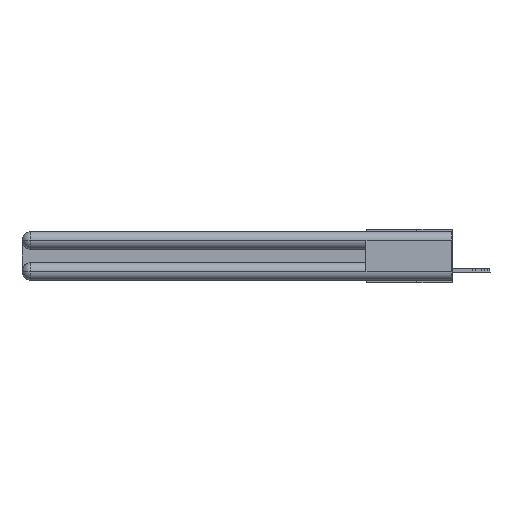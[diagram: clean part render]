
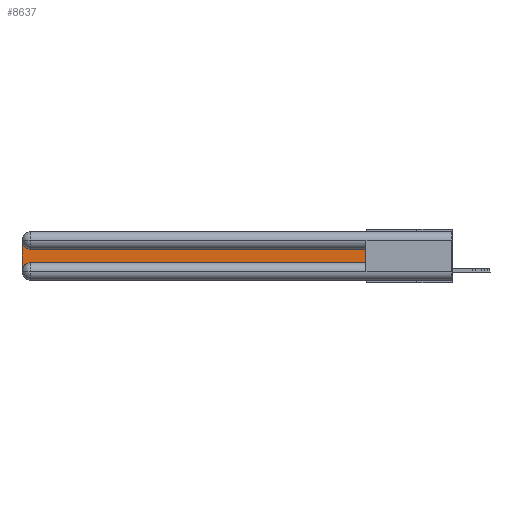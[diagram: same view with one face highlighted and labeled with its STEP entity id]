
A CAD part, left-side view. The second image highlights one B-rep face of the part: STEP entity #8637.
In plain terms, the highlighted planar face has unit normal (-1, 0, 0).
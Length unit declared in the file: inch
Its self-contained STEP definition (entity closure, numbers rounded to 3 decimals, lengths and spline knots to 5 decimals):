
#626 = ORIENTED_EDGE ( 'NONE', *, *, #10922, .T. ) ;
#1539 = DIRECTION ( 'NONE',  ( 1., 0., 0. ) ) ;
#1591 = AXIS2_PLACEMENT_3D ( 'NONE', #20663, #12597, #2594 ) ;
#2594 = DIRECTION ( 'NONE',  ( 0., 0., -1. ) ) ;
#2846 = CARTESIAN_POINT ( 'NONE',  ( 0.075, 0.6, -0.2175 ) ) ;
#2867 = EDGE_CURVE ( 'NONE', #4830, #20696, #9017, .T. ) ;
#3170 = DIRECTION ( 'NONE',  ( 0., 0., -1. ) ) ;
#4822 = VECTOR ( 'NONE', #10806, 39.37008 ) ;
#4830 = VERTEX_POINT ( 'NONE', #29184 ) ;
#4852 = ORIENTED_EDGE ( 'NONE', *, *, #13055, .T. ) ;
#5380 = VECTOR ( 'NONE', #6955, 39.37008 ) ;
#5693 = VERTEX_POINT ( 'NONE', #28996 ) ;
#5864 = VECTOR ( 'NONE', #19027, 39.37008 ) ;
#6955 = DIRECTION ( 'NONE',  ( 0., 0., 1. ) ) ;
#6956 = AXIS2_PLACEMENT_3D ( 'NONE', #14237, #1539, #21978 ) ;
#8501 = CARTESIAN_POINT ( 'NONE',  ( 0.075, 0.6, -0.1225 ) ) ;
#8637 = ADVANCED_FACE ( 'NONE', ( #25916 ), #29512, .F. ) ;
#9017 = LINE ( 'NONE', #8501, #5864 ) ;
#9150 = LINE ( 'NONE', #2846, #4822 ) ;
#9892 = VERTEX_POINT ( 'NONE', #15223 ) ;
#10806 = DIRECTION ( 'NONE',  ( 0., -1., 0. ) ) ;
#10922 = EDGE_CURVE ( 'NONE', #30947, #4830, #32181, .T. ) ;
#11795 = CIRCLE ( 'NONE', #1591, 0.06 ) ;
#12597 = DIRECTION ( 'NONE',  ( 1., 0., 0. ) ) ;
#13055 = EDGE_CURVE ( 'NONE', #20696, #5693, #21182, .T. ) ;
#13077 = EDGE_CURVE ( 'NONE', #26933, #30947, #9150, .T. ) ;
#13784 = ORIENTED_EDGE ( 'NONE', *, *, #2867, .T. ) ;
#14237 = CARTESIAN_POINT ( 'NONE',  ( 0.075, 3., -0.1225 ) ) ;
#14906 = CARTESIAN_POINT ( 'NONE',  ( 0.075, 0.6, -0.2175 ) ) ;
#15223 = CARTESIAN_POINT ( 'NONE',  ( 0.075, 3., -0.2775 ) ) ;
#15667 = CARTESIAN_POINT ( 'NONE',  ( 0.075, 2.94, -0.2175 ) ) ;
#18065 = EDGE_CURVE ( 'NONE', #9892, #26933, #11795, .T. ) ;
#19027 = DIRECTION ( 'NONE',  ( 0., 1., 0. ) ) ;
#20663 = CARTESIAN_POINT ( 'NONE',  ( 0.075, 2.94, -0.2775 ) ) ;
#20696 = VERTEX_POINT ( 'NONE', #24758 ) ;
#21182 = CIRCLE ( 'NONE', #26749, 0.06 ) ;
#21938 = CARTESIAN_POINT ( 'NONE',  ( 0.075, 0.6, -0.2175 ) ) ;
#21978 = DIRECTION ( 'NONE',  ( 0., 0., -1. ) ) ;
#23483 = DIRECTION ( 'NONE',  ( 1., 0., 0. ) ) ;
#24049 = ORIENTED_EDGE ( 'NONE', *, *, #18065, .T. ) ;
#24758 = CARTESIAN_POINT ( 'NONE',  ( 0.075, 2.94, -0.1225 ) ) ;
#24903 = EDGE_LOOP ( 'NONE', ( #13784, #4852, #27246, #24049, #25196, #626 ) ) ;
#25196 = ORIENTED_EDGE ( 'NONE', *, *, #13077, .T. ) ;
#25531 = CARTESIAN_POINT ( 'NONE',  ( 0.075, 3., -0.2175 ) ) ;
#25916 = FACE_OUTER_BOUND ( 'NONE', #24903, .T. ) ;
#26749 = AXIS2_PLACEMENT_3D ( 'NONE', #31023, #23483, #3170 ) ;
#26933 = VERTEX_POINT ( 'NONE', #15667 ) ;
#27246 = ORIENTED_EDGE ( 'NONE', *, *, #28462, .T. ) ;
#28284 = DIRECTION ( 'NONE',  ( 0., 0., -1. ) ) ;
#28462 = EDGE_CURVE ( 'NONE', #5693, #9892, #32276, .T. ) ;
#28996 = CARTESIAN_POINT ( 'NONE',  ( 0.075, 3., -0.0625 ) ) ;
#29184 = CARTESIAN_POINT ( 'NONE',  ( 0.075, 0.6, -0.1225 ) ) ;
#29512 = PLANE ( 'NONE',  #6956 ) ;
#30947 = VERTEX_POINT ( 'NONE', #14906 ) ;
#31023 = CARTESIAN_POINT ( 'NONE',  ( 0.075, 2.94, -0.0625 ) ) ;
#32181 = LINE ( 'NONE', #21938, #5380 ) ;
#32276 = LINE ( 'NONE', #25531, #33072 ) ;
#33072 = VECTOR ( 'NONE', #28284, 39.37008 ) ;
